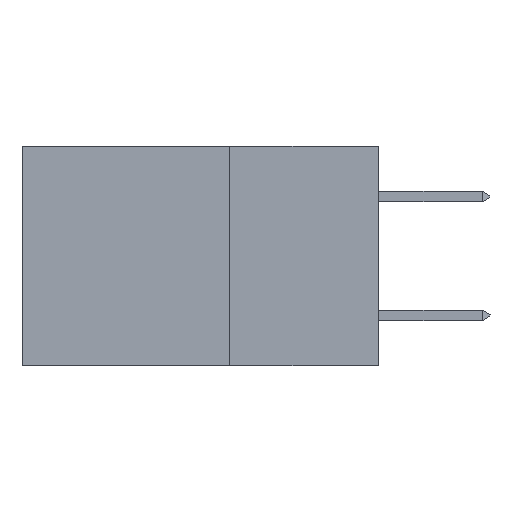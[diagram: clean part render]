
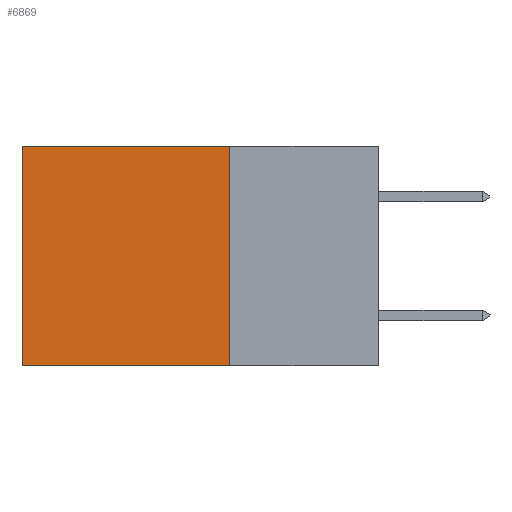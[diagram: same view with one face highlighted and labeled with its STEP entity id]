
A CAD part, left-side view. The second image highlights one B-rep face of the part: STEP entity #6869.
In plain terms, the highlighted planar face has unit normal (-1, 0, 0).
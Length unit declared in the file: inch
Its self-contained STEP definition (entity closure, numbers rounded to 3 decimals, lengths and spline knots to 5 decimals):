
#201 = ORIENTED_EDGE ( 'NONE', *, *, #6815, .T. ) ;
#474 = VERTEX_POINT ( 'NONE', #6677 ) ;
#594 = CARTESIAN_POINT ( 'NONE',  ( 0.298, 0.25, -0.37 ) ) ;
#919 = LINE ( 'NONE', #2298, #12590 ) ;
#1041 = DIRECTION ( 'NONE',  ( 0., 0., -1. ) ) ;
#1195 = DIRECTION ( 'NONE',  ( 0., 0., -1. ) ) ;
#1719 = CARTESIAN_POINT ( 'NONE',  ( 0.298, 0.25, 0. ) ) ;
#2139 = LINE ( 'NONE', #10295, #4256 ) ;
#2151 = VERTEX_POINT ( 'NONE', #5413 ) ;
#2160 = ORIENTED_EDGE ( 'NONE', *, *, #13460, .F. ) ;
#2298 = CARTESIAN_POINT ( 'NONE',  ( 0.298, 0.6, 0. ) ) ;
#3283 = AXIS2_PLACEMENT_3D ( 'NONE', #12601, #5800, #10845 ) ;
#3301 = VECTOR ( 'NONE', #9615, 39.37008 ) ;
#3656 = LINE ( 'NONE', #594, #3301 ) ;
#3871 = DIRECTION ( 'NONE',  ( 0., 1., 0. ) ) ;
#4256 = VECTOR ( 'NONE', #1195, 39.37008 ) ;
#4962 = LINE ( 'NONE', #13690, #11726 ) ;
#5413 = CARTESIAN_POINT ( 'NONE',  ( 0.298, 0.25, -0.37 ) ) ;
#5786 = EDGE_LOOP ( 'NONE', ( #6036, #12325, #2160, #201 ) ) ;
#5800 = DIRECTION ( 'NONE',  ( 1., 0., 0. ) ) ;
#6036 = ORIENTED_EDGE ( 'NONE', *, *, #8038, .T. ) ;
#6353 = VERTEX_POINT ( 'NONE', #12848 ) ;
#6677 = CARTESIAN_POINT ( 'NONE',  ( 0.298, 0.6, 0. ) ) ;
#6815 = EDGE_CURVE ( 'NONE', #10126, #474, #4962, .T. ) ;
#6869 = ADVANCED_FACE ( 'NONE', ( #7959 ), #11446, .F. ) ;
#7959 = FACE_OUTER_BOUND ( 'NONE', #5786, .T. ) ;
#8038 = EDGE_CURVE ( 'NONE', #474, #6353, #919, .T. ) ;
#9556 = EDGE_CURVE ( 'NONE', #2151, #6353, #3656, .T. ) ;
#9615 = DIRECTION ( 'NONE',  ( 0., 1., 0. ) ) ;
#10126 = VERTEX_POINT ( 'NONE', #1719 ) ;
#10295 = CARTESIAN_POINT ( 'NONE',  ( 0.298, 0.25, 0. ) ) ;
#10845 = DIRECTION ( 'NONE',  ( 0., 0., -1. ) ) ;
#11446 = PLANE ( 'NONE',  #3283 ) ;
#11726 = VECTOR ( 'NONE', #3871, 39.37008 ) ;
#12325 = ORIENTED_EDGE ( 'NONE', *, *, #9556, .F. ) ;
#12590 = VECTOR ( 'NONE', #1041, 39.37008 ) ;
#12601 = CARTESIAN_POINT ( 'NONE',  ( 0.298, 0.25, 0. ) ) ;
#12848 = CARTESIAN_POINT ( 'NONE',  ( 0.298, 0.6, -0.37 ) ) ;
#13460 = EDGE_CURVE ( 'NONE', #10126, #2151, #2139, .T. ) ;
#13690 = CARTESIAN_POINT ( 'NONE',  ( 0.298, 0.25, 0. ) ) ;
